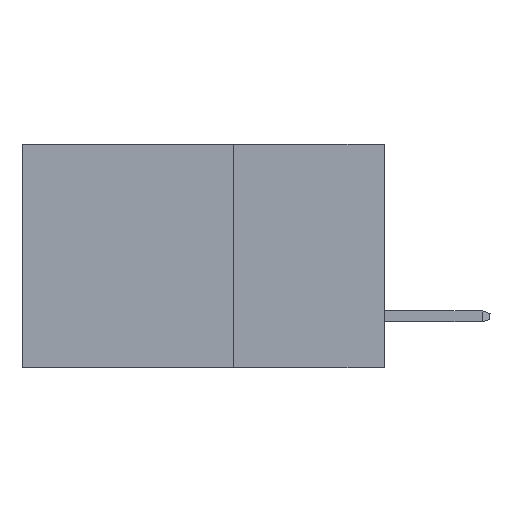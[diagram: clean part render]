
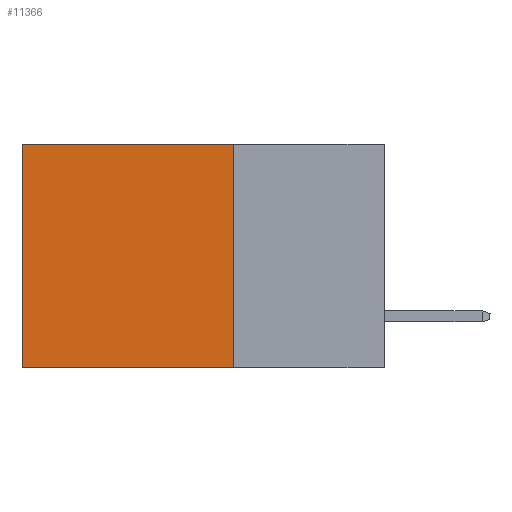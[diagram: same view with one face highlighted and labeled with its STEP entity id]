
A CAD part, left-side view. The second image highlights one B-rep face of the part: STEP entity #11366.
In plain terms, the highlighted planar face has unit normal (-1, 0, 0).
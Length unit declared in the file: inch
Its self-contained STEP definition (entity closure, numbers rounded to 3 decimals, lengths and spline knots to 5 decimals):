
#476 = DIRECTION ( 'NONE',  ( 0., 0., -1. ) ) ;
#509 = CARTESIAN_POINT ( 'NONE',  ( 0.298, 0.25, 0. ) ) ;
#1206 = VERTEX_POINT ( 'NONE', #3993 ) ;
#1391 = VERTEX_POINT ( 'NONE', #6579 ) ;
#1417 = DIRECTION ( 'NONE',  ( 0., 0., -1. ) ) ;
#1847 = LINE ( 'NONE', #9373, #8884 ) ;
#2617 = EDGE_CURVE ( 'NONE', #1206, #11153, #5722, .T. ) ;
#2908 = EDGE_CURVE ( 'NONE', #1391, #5673, #3875, .T. ) ;
#2936 = EDGE_CURVE ( 'NONE', #11153, #5673, #3175, .T. ) ;
#3175 = LINE ( 'NONE', #10345, #11053 ) ;
#3360 = ORIENTED_EDGE ( 'NONE', *, *, #2936, .T. ) ;
#3509 = CARTESIAN_POINT ( 'NONE',  ( 0.298, 0.6, -0.37 ) ) ;
#3875 = LINE ( 'NONE', #9315, #4720 ) ;
#3993 = CARTESIAN_POINT ( 'NONE',  ( 0.298, 0.25, 0. ) ) ;
#4720 = VECTOR ( 'NONE', #8505, 39.37008 ) ;
#5673 = VERTEX_POINT ( 'NONE', #3509 ) ;
#5722 = LINE ( 'NONE', #509, #9811 ) ;
#6027 = ORIENTED_EDGE ( 'NONE', *, *, #2617, .T. ) ;
#6384 = EDGE_CURVE ( 'NONE', #1206, #1391, #1847, .T. ) ;
#6579 = CARTESIAN_POINT ( 'NONE',  ( 0.298, 0.25, -0.37 ) ) ;
#6808 = EDGE_LOOP ( 'NONE', ( #3360, #11023, #6833, #6027 ) ) ;
#6833 = ORIENTED_EDGE ( 'NONE', *, *, #6384, .F. ) ;
#6911 = FACE_OUTER_BOUND ( 'NONE', #6808, .T. ) ;
#7139 = AXIS2_PLACEMENT_3D ( 'NONE', #10576, #9557, #1417 ) ;
#7327 = CARTESIAN_POINT ( 'NONE',  ( 0.298, 0.6, 0. ) ) ;
#8281 = PLANE ( 'NONE',  #7139 ) ;
#8456 = DIRECTION ( 'NONE',  ( 0., 1., 0. ) ) ;
#8505 = DIRECTION ( 'NONE',  ( 0., 1., 0. ) ) ;
#8523 = DIRECTION ( 'NONE',  ( 0., 0., -1. ) ) ;
#8884 = VECTOR ( 'NONE', #8523, 39.37008 ) ;
#9315 = CARTESIAN_POINT ( 'NONE',  ( 0.298, 0.25, -0.37 ) ) ;
#9373 = CARTESIAN_POINT ( 'NONE',  ( 0.298, 0.25, 0. ) ) ;
#9557 = DIRECTION ( 'NONE',  ( 1., 0., 0. ) ) ;
#9811 = VECTOR ( 'NONE', #8456, 39.37008 ) ;
#10345 = CARTESIAN_POINT ( 'NONE',  ( 0.298, 0.6, 0. ) ) ;
#10576 = CARTESIAN_POINT ( 'NONE',  ( 0.298, 0.25, 0. ) ) ;
#11023 = ORIENTED_EDGE ( 'NONE', *, *, #2908, .F. ) ;
#11053 = VECTOR ( 'NONE', #476, 39.37008 ) ;
#11153 = VERTEX_POINT ( 'NONE', #7327 ) ;
#11366 = ADVANCED_FACE ( 'NONE', ( #6911 ), #8281, .F. ) ;
